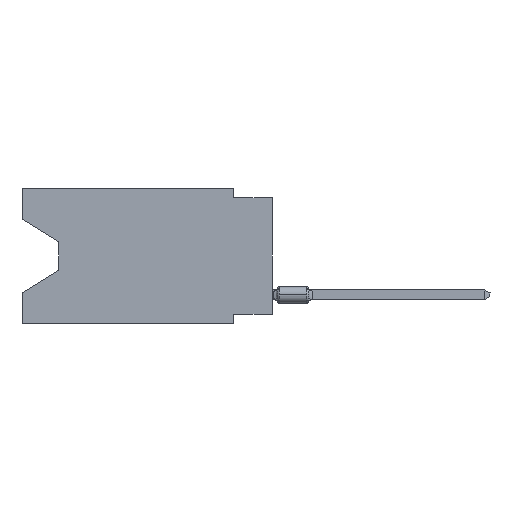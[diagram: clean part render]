
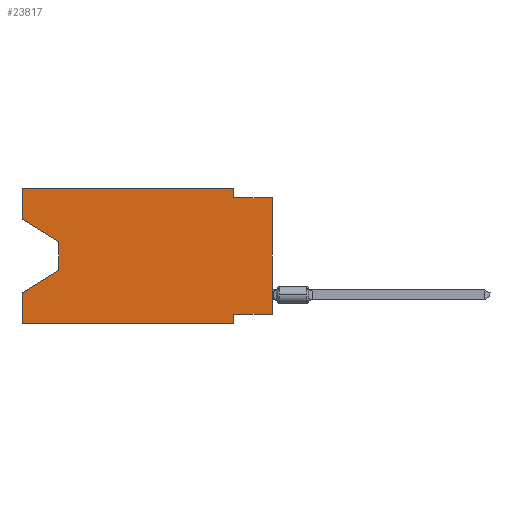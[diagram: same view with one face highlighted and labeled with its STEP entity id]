
A CAD part, left-side view. The second image highlights one B-rep face of the part: STEP entity #23817.
In plain terms, the highlighted planar face has unit normal (-1, 0, 0).
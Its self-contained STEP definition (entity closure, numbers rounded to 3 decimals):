
#957 = ORIENTED_EDGE ( 'NONE', *, *, #76661, .F. ) ;
#1441 = CARTESIAN_POINT ( 'NONE',  ( 0., 16.383, -2.038 ) ) ;
#1620 = DIRECTION ( 'NONE',  ( 0., 0., 1. ) ) ;
#1783 = EDGE_CURVE ( 'NONE', #69148, #49466, #69862, .T. ) ;
#2616 = ORIENTED_EDGE ( 'NONE', *, *, #52123, .F. ) ;
#3117 = EDGE_CURVE ( 'NONE', #84314, #79028, #68699, .T. ) ;
#3389 = CARTESIAN_POINT ( 'NONE',  ( 0., 2.54, 0. ) ) ;
#3894 = CARTESIAN_POINT ( 'NONE',  ( 0., 13.97, -3.505 ) ) ;
#6151 = AXIS2_PLACEMENT_3D ( 'NONE', #50744, #43262, #80977 ) ;
#6707 = EDGE_CURVE ( 'NONE', #30579, #97509, #50196, .T. ) ;
#7983 = CARTESIAN_POINT ( 'NONE',  ( 0., 16.383, -8.89 ) ) ;
#11362 = LINE ( 'NONE', #43151, #51893 ) ;
#11834 = VECTOR ( 'NONE', #87771, 1000. ) ;
#12545 = DIRECTION ( 'NONE',  ( 0., 1., 0. ) ) ;
#14043 = LINE ( 'NONE', #43851, #88403 ) ;
#14955 = DIRECTION ( 'NONE',  ( 0., -1., 0. ) ) ;
#15572 = VECTOR ( 'NONE', #77850, 1000. ) ;
#16013 = LINE ( 'NONE', #69626, #44843 ) ;
#17307 = LINE ( 'NONE', #1441, #15572 ) ;
#17354 = CARTESIAN_POINT ( 'NONE',  ( 0., 0., -0.635 ) ) ;
#18794 = LINE ( 'NONE', #3894, #11834 ) ;
#21838 = EDGE_CURVE ( 'NONE', #30579, #66741, #17307, .T. ) ;
#23534 = DIRECTION ( 'NONE',  ( 0., 0., -1. ) ) ;
#23817 = ADVANCED_FACE ( 'NONE', ( #89410 ), #90854, .F. ) ;
#24953 = ORIENTED_EDGE ( 'NONE', *, *, #82802, .T. ) ;
#25186 = EDGE_CURVE ( 'NONE', #66741, #69148, #18794, .T. ) ;
#26291 = DIRECTION ( 'NONE',  ( 0., -1., 0. ) ) ;
#27443 = LINE ( 'NONE', #82026, #62232 ) ;
#29888 = CARTESIAN_POINT ( 'NONE',  ( 0., 16.383, -8.89 ) ) ;
#30579 = VERTEX_POINT ( 'NONE', #51624 ) ;
#32791 = VERTEX_POINT ( 'NONE', #67855 ) ;
#34283 = CARTESIAN_POINT ( 'NONE',  ( 0., 13.97, -3.505 ) ) ;
#39533 = EDGE_CURVE ( 'NONE', #97509, #45614, #78509, .T. ) ;
#39657 = ORIENTED_EDGE ( 'NONE', *, *, #47835, .F. ) ;
#39962 = ORIENTED_EDGE ( 'NONE', *, *, #3117, .F. ) ;
#40872 = VECTOR ( 'NONE', #94016, 1000. ) ;
#41525 = DIRECTION ( 'NONE',  ( 0., 0.855, -0.519 ) ) ;
#42001 = CARTESIAN_POINT ( 'NONE',  ( 0., 13.97, -5.385 ) ) ;
#43151 = CARTESIAN_POINT ( 'NONE',  ( 0., 0., -0.635 ) ) ;
#43262 = DIRECTION ( 'NONE',  ( 1., 0., 0. ) ) ;
#43698 = VECTOR ( 'NONE', #14955, 1000. ) ;
#43777 = ORIENTED_EDGE ( 'NONE', *, *, #39533, .F. ) ;
#43851 = CARTESIAN_POINT ( 'NONE',  ( 0., 2.54, 0. ) ) ;
#44843 = VECTOR ( 'NONE', #1620, 1000. ) ;
#45614 = VERTEX_POINT ( 'NONE', #3389 ) ;
#46572 = ORIENTED_EDGE ( 'NONE', *, *, #21838, .T. ) ;
#47274 = CARTESIAN_POINT ( 'NONE',  ( 0., 16.383, 0. ) ) ;
#47835 = EDGE_CURVE ( 'NONE', #32791, #84314, #27443, .T. ) ;
#48878 = LINE ( 'NONE', #92561, #40872 ) ;
#49466 = VERTEX_POINT ( 'NONE', #72200 ) ;
#50062 = ORIENTED_EDGE ( 'NONE', *, *, #61083, .T. ) ;
#50196 = LINE ( 'NONE', #95826, #58519 ) ;
#50393 = ORIENTED_EDGE ( 'NONE', *, *, #25186, .T. ) ;
#50744 = CARTESIAN_POINT ( 'NONE',  ( 0., 16.383, 0. ) ) ;
#51624 = CARTESIAN_POINT ( 'NONE',  ( 0., 16.383, -2.038 ) ) ;
#51893 = VECTOR ( 'NONE', #26291, 1000. ) ;
#52123 = EDGE_CURVE ( 'NONE', #93330, #72564, #11362, .T. ) ;
#56204 = CARTESIAN_POINT ( 'NONE',  ( 0., 2.54, -8.89 ) ) ;
#58519 = VECTOR ( 'NONE', #80445, 1000. ) ;
#59051 = CARTESIAN_POINT ( 'NONE',  ( 0., 2.54, -0.635 ) ) ;
#61083 = EDGE_CURVE ( 'NONE', #90177, #79028, #61114, .T. ) ;
#61114 = LINE ( 'NONE', #29888, #43698 ) ;
#61264 = CARTESIAN_POINT ( 'NONE',  ( 0., 2.54, -8.89 ) ) ;
#62232 = VECTOR ( 'NONE', #12545, 1000. ) ;
#63540 = ORIENTED_EDGE ( 'NONE', *, *, #1783, .T. ) ;
#63695 = EDGE_LOOP ( 'NONE', ( #46572, #50393, #63540, #83199, #50062, #39962, #39657, #24953, #2616, #957, #43777, #85090 ) ) ;
#65824 = CARTESIAN_POINT ( 'NONE',  ( 0., 2.54, -8.255 ) ) ;
#66741 = VERTEX_POINT ( 'NONE', #34283 ) ;
#67510 = VECTOR ( 'NONE', #41525, 1000. ) ;
#67855 = CARTESIAN_POINT ( 'NONE',  ( 0., 0., -8.255 ) ) ;
#68699 = LINE ( 'NONE', #61264, #91285 ) ;
#69148 = VERTEX_POINT ( 'NONE', #42001 ) ;
#69626 = CARTESIAN_POINT ( 'NONE',  ( 0., 0., 0. ) ) ;
#69862 = LINE ( 'NONE', #88682, #67510 ) ;
#72200 = CARTESIAN_POINT ( 'NONE',  ( 0., 16.383, -6.852 ) ) ;
#72564 = VERTEX_POINT ( 'NONE', #17354 ) ;
#76661 = EDGE_CURVE ( 'NONE', #45614, #93330, #14043, .T. ) ;
#77850 = DIRECTION ( 'NONE',  ( 0., -0.855, -0.519 ) ) ;
#78509 = LINE ( 'NONE', #47274, #84543 ) ;
#79028 = VERTEX_POINT ( 'NONE', #56204 ) ;
#80445 = DIRECTION ( 'NONE',  ( 0., 0., 1. ) ) ;
#80977 = DIRECTION ( 'NONE',  ( 0., 0., -1. ) ) ;
#82026 = CARTESIAN_POINT ( 'NONE',  ( 0., 0., -8.255 ) ) ;
#82802 = EDGE_CURVE ( 'NONE', #32791, #72564, #16013, .T. ) ;
#83199 = ORIENTED_EDGE ( 'NONE', *, *, #92137, .F. ) ;
#84314 = VERTEX_POINT ( 'NONE', #65824 ) ;
#84543 = VECTOR ( 'NONE', #92924, 1000. ) ;
#85090 = ORIENTED_EDGE ( 'NONE', *, *, #6707, .F. ) ;
#87771 = DIRECTION ( 'NONE',  ( 0., 0., -1. ) ) ;
#88016 = DIRECTION ( 'NONE',  ( 0., 0., -1. ) ) ;
#88403 = VECTOR ( 'NONE', #88016, 1000. ) ;
#88682 = CARTESIAN_POINT ( 'NONE',  ( 0., 13.97, -5.385 ) ) ;
#89410 = FACE_OUTER_BOUND ( 'NONE', #63695, .T. ) ;
#90177 = VERTEX_POINT ( 'NONE', #7983 ) ;
#90854 = PLANE ( 'NONE',  #6151 ) ;
#91285 = VECTOR ( 'NONE', #23534, 1000. ) ;
#92137 = EDGE_CURVE ( 'NONE', #90177, #49466, #48878, .T. ) ;
#92561 = CARTESIAN_POINT ( 'NONE',  ( 0., 16.383, 0. ) ) ;
#92924 = DIRECTION ( 'NONE',  ( 0., -1., 0. ) ) ;
#93330 = VERTEX_POINT ( 'NONE', #59051 ) ;
#94016 = DIRECTION ( 'NONE',  ( 0., 0., 1. ) ) ;
#95082 = CARTESIAN_POINT ( 'NONE',  ( 0., 16.383, 0. ) ) ;
#95826 = CARTESIAN_POINT ( 'NONE',  ( 0., 16.383, 0. ) ) ;
#97509 = VERTEX_POINT ( 'NONE', #95082 ) ;
